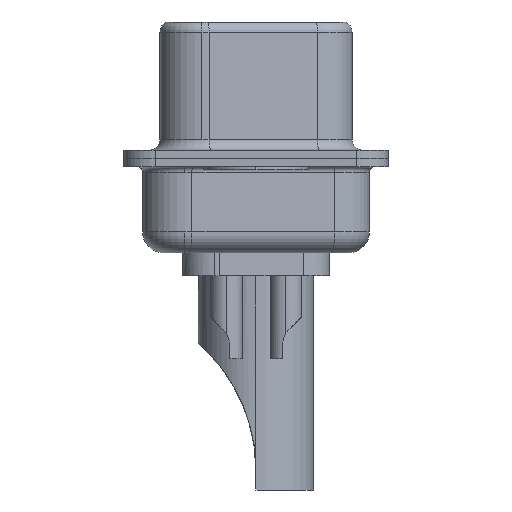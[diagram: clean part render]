
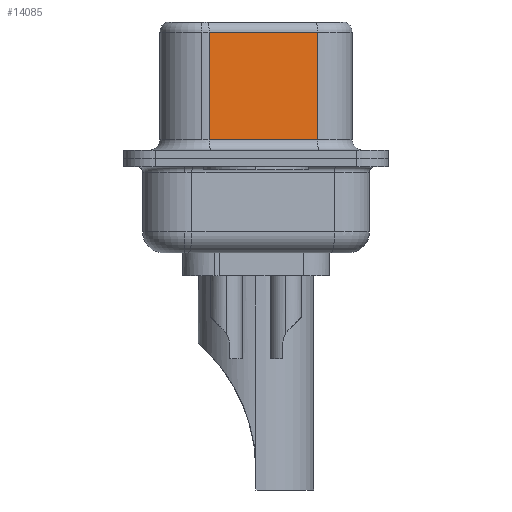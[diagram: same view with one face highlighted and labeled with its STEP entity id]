
A CAD part, left-side view. The second image highlights one B-rep face of the part: STEP entity #14085.
In plain terms, the highlighted planar face has unit normal (-0.985, -0.174, 0).
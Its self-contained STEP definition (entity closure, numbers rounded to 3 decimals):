
#222 = ORIENTED_EDGE ( 'NONE', *, *, #4508, .T. ) ;
#313 = VERTEX_POINT ( 'NONE', #7274 ) ;
#605 = DIRECTION ( 'NONE',  ( -0.174, 0.985, 0. ) ) ;
#835 = DIRECTION ( 'NONE',  ( -0.174, 0.985, 0. ) ) ;
#1273 = DIRECTION ( 'NONE',  ( 0., 0., -1. ) ) ;
#1909 = DIRECTION ( 'NONE',  ( 0.174, -0.985, 0. ) ) ;
#1927 = LINE ( 'NONE', #10127, #8497 ) ;
#1928 = EDGE_CURVE ( 'NONE', #13183, #313, #9564, .T. ) ;
#1959 = VECTOR ( 'NONE', #11669, 1000. ) ;
#3368 = EDGE_CURVE ( 'NONE', #9580, #12861, #12805, .T. ) ;
#3445 = EDGE_CURVE ( 'NONE', #13183, #12861, #5638, .T. ) ;
#4508 = EDGE_CURVE ( 'NONE', #313, #9580, #1927, .T. ) ;
#4577 = CARTESIAN_POINT ( 'NONE',  ( 4.565, -2.927, 0.9 ) ) ;
#4665 = CARTESIAN_POINT ( 'NONE',  ( 4.565, -2.927, 6.52 ) ) ;
#4927 = CARTESIAN_POINT ( 'NONE',  ( 4.565, -2.927, 6.02 ) ) ;
#5271 = AXIS2_PLACEMENT_3D ( 'NONE', #5584, #12807, #605 ) ;
#5341 = CARTESIAN_POINT ( 'NONE',  ( 4.565, -2.927, 0.9 ) ) ;
#5584 = CARTESIAN_POINT ( 'NONE',  ( 4.565, -2.927, 6.52 ) ) ;
#5638 = LINE ( 'NONE', #4665, #1959 ) ;
#6291 = VECTOR ( 'NONE', #835, 1000. ) ;
#6442 = ORIENTED_EDGE ( 'NONE', *, *, #3368, .T. ) ;
#7190 = ORIENTED_EDGE ( 'NONE', *, *, #1928, .T. ) ;
#7274 = CARTESIAN_POINT ( 'NONE',  ( 3.655, 2.233, 6.02 ) ) ;
#7734 = CARTESIAN_POINT ( 'NONE',  ( 3.655, 2.233, 0.9 ) ) ;
#8497 = VECTOR ( 'NONE', #1273, 1000. ) ;
#9564 = LINE ( 'NONE', #4927, #6291 ) ;
#9580 = VERTEX_POINT ( 'NONE', #7734 ) ;
#9661 = VECTOR ( 'NONE', #1909, 1000. ) ;
#10127 = CARTESIAN_POINT ( 'NONE',  ( 3.655, 2.233, 6.52 ) ) ;
#10838 = ORIENTED_EDGE ( 'NONE', *, *, #3445, .F. ) ;
#11036 = CARTESIAN_POINT ( 'NONE',  ( 4.565, -2.927, 6.02 ) ) ;
#11669 = DIRECTION ( 'NONE',  ( 0., 0., -1. ) ) ;
#12805 = LINE ( 'NONE', #5341, #9661 ) ;
#12807 = DIRECTION ( 'NONE',  ( 0.985, 0.174, 0. ) ) ;
#12861 = VERTEX_POINT ( 'NONE', #4577 ) ;
#13183 = VERTEX_POINT ( 'NONE', #11036 ) ;
#14085 = ADVANCED_FACE ( 'NONE', ( #14239 ), #14956, .F. ) ;
#14239 = FACE_OUTER_BOUND ( 'NONE', #14269, .T. ) ;
#14269 = EDGE_LOOP ( 'NONE', ( #10838, #7190, #222, #6442 ) ) ;
#14956 = PLANE ( 'NONE',  #5271 ) ;
